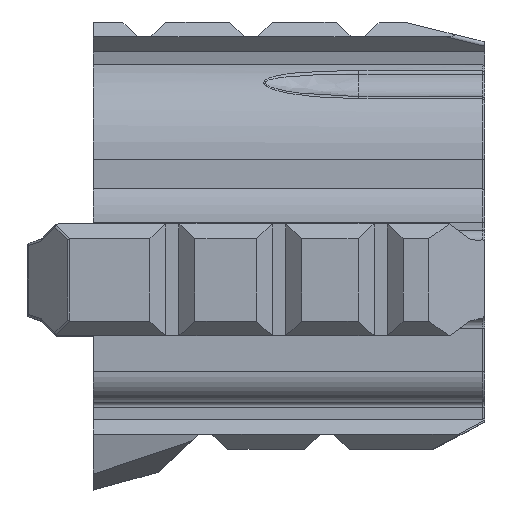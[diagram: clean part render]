
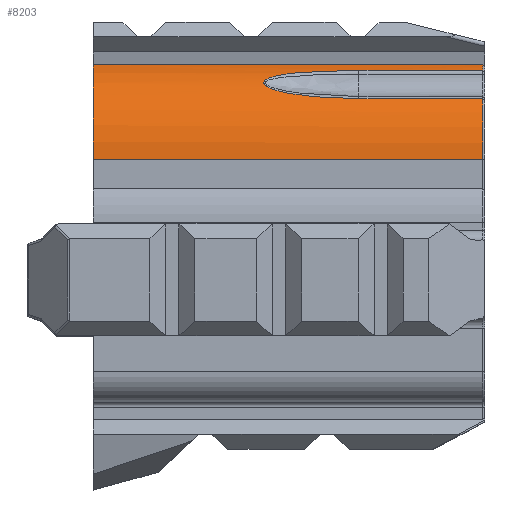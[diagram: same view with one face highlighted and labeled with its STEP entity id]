
A CAD part, top view. The second image highlights one B-rep face of the part: STEP entity #8203.
In plain terms, the highlighted cylindrical face has radius 20.1 mm (diameter 40.2 mm), a partial arc.
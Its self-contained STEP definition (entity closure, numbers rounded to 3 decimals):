
#185 = CYLINDRICAL_SURFACE ( 'NONE', #3875, 20.1 ) ;
#345 = ORIENTED_EDGE ( 'NONE', *, *, #7756, .F. ) ;
#426 = CIRCLE ( 'NONE', #1866, 20.1 ) ;
#433 = VECTOR ( 'NONE', #7498, 1000. ) ;
#647 = DIRECTION ( 'NONE',  ( 0., 0., -1. ) ) ;
#737 = CARTESIAN_POINT ( 'NONE',  ( 54.049, 64.619, 11.305 ) ) ;
#739 = ORIENTED_EDGE ( 'NONE', *, *, #1415, .F. ) ;
#896 = CARTESIAN_POINT ( 'NONE',  ( 45.726, 61.611, 15.192 ) ) ;
#1023 = LINE ( 'NONE', #1203, #4756 ) ;
#1192 = CARTESIAN_POINT ( 'NONE',  ( 11.678, 65.991, 8.545 ) ) ;
#1203 = CARTESIAN_POINT ( 'NONE',  ( -12.072, 47.361, 21.1 ) ) ;
#1415 = EDGE_CURVE ( 'NONE', #3280, #4947, #5673, .T. ) ;
#1496 = CARTESIAN_POINT ( 'NONE',  ( -12.072, 47.361, 1. ) ) ;
#1507 = EDGE_CURVE ( 'NONE', #3093, #2727, #7244, .T. ) ;
#1795 = ORIENTED_EDGE ( 'NONE', *, *, #4805, .F. ) ;
#1866 = AXIS2_PLACEMENT_3D ( 'NONE', #8350, #5467, #3994 ) ;
#2140 = CARTESIAN_POINT ( 'NONE',  ( 45.675, 63.116, 13.486 ) ) ;
#2201 = CARTESIAN_POINT ( 'NONE',  ( 55.931, 64.737, 11.106 ) ) ;
#2266 = CARTESIAN_POINT ( 'NONE',  ( 62.068, 64.924, 10.776 ) ) ;
#2270 = EDGE_CURVE ( 'NONE', #3624, #3998, #8674, .T. ) ;
#2409 = FACE_OUTER_BOUND ( 'NONE', #3690, .T. ) ;
#2525 = LINE ( 'NONE', #3881, #8267 ) ;
#2727 = VERTEX_POINT ( 'NONE', #8306 ) ;
#2881 = CARTESIAN_POINT ( 'NONE',  ( 63.96, 64.924, 10.776 ) ) ;
#2926 = CARTESIAN_POINT ( 'NONE',  ( 63.96, 64.924, 10.776 ) ) ;
#2935 = CARTESIAN_POINT ( 'NONE',  ( 190.555, 64.924, 10.776 ) ) ;
#2950 = LINE ( 'NONE', #2935, #9059 ) ;
#3042 = CARTESIAN_POINT ( 'NONE',  ( 55.12, 59.523, 17.02 ) ) ;
#3093 = VERTEX_POINT ( 'NONE', #1192 ) ;
#3280 = VERTEX_POINT ( 'NONE', #2881 ) ;
#3566 = CARTESIAN_POINT ( 'NONE',  ( 45.302, 62.776, 13.902 ) ) ;
#3582 = ORIENTED_EDGE ( 'NONE', *, *, #4268, .F. ) ;
#3624 = VERTEX_POINT ( 'NONE', #5366 ) ;
#3634 = CARTESIAN_POINT ( 'NONE',  ( 88.3, 64.924, 10.776 ) ) ;
#3672 = CARTESIAN_POINT ( 'NONE',  ( 47.724, 63.86, 12.49 ) ) ;
#3690 = EDGE_LOOP ( 'NONE', ( #6662, #1795, #739, #345, #7715, #3582, #6290, #7940 ) ) ;
#3762 = DIRECTION ( 'NONE',  ( 1., 0., 0. ) ) ;
#3812 = CARTESIAN_POINT ( 'NONE',  ( 46.878, 61.167, 15.61 ) ) ;
#3821 = VERTEX_POINT ( 'NONE', #4080 ) ;
#3875 = AXIS2_PLACEMENT_3D ( 'NONE', #1496, #4873, #647 ) ;
#3881 = CARTESIAN_POINT ( 'NONE',  ( 190.555, 59.295, 17.174 ) ) ;
#3994 = DIRECTION ( 'NONE',  ( 0., 0., 1. ) ) ;
#3998 = VERTEX_POINT ( 'NONE', #6420 ) ;
#4080 = CARTESIAN_POINT ( 'NONE',  ( 88.3, 65.991, 8.545 ) ) ;
#4268 = EDGE_CURVE ( 'NONE', #3093, #3821, #7176, .T. ) ;
#4432 = CARTESIAN_POINT ( 'NONE',  ( 11.678, 47.361, 1. ) ) ;
#4756 = VECTOR ( 'NONE', #8234, 1000. ) ;
#4793 = CARTESIAN_POINT ( 'NONE',  ( 63.96, 59.295, 17.174 ) ) ;
#4805 = EDGE_CURVE ( 'NONE', #4947, #3624, #2525, .T. ) ;
#4814 = DIRECTION ( 'NONE',  ( 1., 0., 0. ) ) ;
#4873 = DIRECTION ( 'NONE',  ( 1., 0., 0. ) ) ;
#4947 = VERTEX_POINT ( 'NONE', #4793 ) ;
#5132 = DIRECTION ( 'NONE',  ( 0., 0., -1. ) ) ;
#5366 = CARTESIAN_POINT ( 'NONE',  ( 88.3, 59.295, 17.174 ) ) ;
#5467 = DIRECTION ( 'NONE',  ( 1., 0., 0. ) ) ;
#5673 = B_SPLINE_CURVE_WITH_KNOTS ( 'NONE', 3,
 ( #2926, #2266, #5774, #2201, #737, #6360, #7128, #3672, #8618, #2140, #3566, #5924, #896, #3812, #5894, #8744, #3042, #6587, #5864 ),
 .UNSPECIFIED., .F., .F.,
 ( 4, 1, 1, 1, 1, 1, 1, 1, 1, 1, 1, 1, 1, 1, 1, 1, 4 ),
 ( 0., 0.143, 0.214, 0.25, 0.286, 0.357, 0.429, 0.452, 0.476, 0.488, 0.5, 0.524, 0.571, 0.595, 0.619, 0.714, 1. ),
 .UNSPECIFIED. ) ;
#5774 = CARTESIAN_POINT ( 'NONE',  ( 59.228, 64.88, 10.855 ) ) ;
#5864 = CARTESIAN_POINT ( 'NONE',  ( 63.96, 59.295, 17.174 ) ) ;
#5878 = VERTEX_POINT ( 'NONE', #3634 ) ;
#5894 = CARTESIAN_POINT ( 'NONE',  ( 48.041, 60.807, 15.942 ) ) ;
#5924 = CARTESIAN_POINT ( 'NONE',  ( 45.137, 62.339, 14.412 ) ) ;
#6290 = ORIENTED_EDGE ( 'NONE', *, *, #1507, .T. ) ;
#6360 = CARTESIAN_POINT ( 'NONE',  ( 52.173, 64.474, 11.546 ) ) ;
#6420 = CARTESIAN_POINT ( 'NONE',  ( 88.3, 47.361, 21.1 ) ) ;
#6470 = DIRECTION ( 'NONE',  ( -1., 0., 0. ) ) ;
#6587 = CARTESIAN_POINT ( 'NONE',  ( 60.176, 59.295, 17.174 ) ) ;
#6588 = EDGE_CURVE ( 'NONE', #3821, #5878, #426, .T. ) ;
#6603 = AXIS2_PLACEMENT_3D ( 'NONE', #6856, #4814, #8221 ) ;
#6662 = ORIENTED_EDGE ( 'NONE', *, *, #2270, .F. ) ;
#6856 = CARTESIAN_POINT ( 'NONE',  ( 88.3, 47.361, 1. ) ) ;
#7128 = CARTESIAN_POINT ( 'NONE',  ( 49.862, 64.227, 11.94 ) ) ;
#7176 = LINE ( 'NONE', #8977, #433 ) ;
#7244 = CIRCLE ( 'NONE', #8325, 20.1 ) ;
#7498 = DIRECTION ( 'NONE',  ( 1., 0., 0. ) ) ;
#7715 = ORIENTED_EDGE ( 'NONE', *, *, #6588, .F. ) ;
#7756 = EDGE_CURVE ( 'NONE', #5878, #3280, #2950, .T. ) ;
#7940 = ORIENTED_EDGE ( 'NONE', *, *, #8830, .F. ) ;
#8077 = DIRECTION ( 'NONE',  ( 1., 0., 0. ) ) ;
#8203 = ADVANCED_FACE ( 'NONE', ( #2409 ), #185, .T. ) ;
#8221 = DIRECTION ( 'NONE',  ( 0., 0., 1. ) ) ;
#8234 = DIRECTION ( 'NONE',  ( -1., 0., 0. ) ) ;
#8267 = VECTOR ( 'NONE', #8077, 1000. ) ;
#8306 = CARTESIAN_POINT ( 'NONE',  ( 11.678, 47.361, 21.1 ) ) ;
#8325 = AXIS2_PLACEMENT_3D ( 'NONE', #4432, #3762, #5132 ) ;
#8350 = CARTESIAN_POINT ( 'NONE',  ( 88.3, 47.361, 1. ) ) ;
#8618 = CARTESIAN_POINT ( 'NONE',  ( 46.315, 63.423, 13.087 ) ) ;
#8674 = CIRCLE ( 'NONE', #6603, 20.1 ) ;
#8744 = CARTESIAN_POINT ( 'NONE',  ( 49.861, 60.363, 16.333 ) ) ;
#8830 = EDGE_CURVE ( 'NONE', #3998, #2727, #1023, .T. ) ;
#8977 = CARTESIAN_POINT ( 'NONE',  ( -12.072, 65.991, 8.545 ) ) ;
#9059 = VECTOR ( 'NONE', #6470, 1000. ) ;
